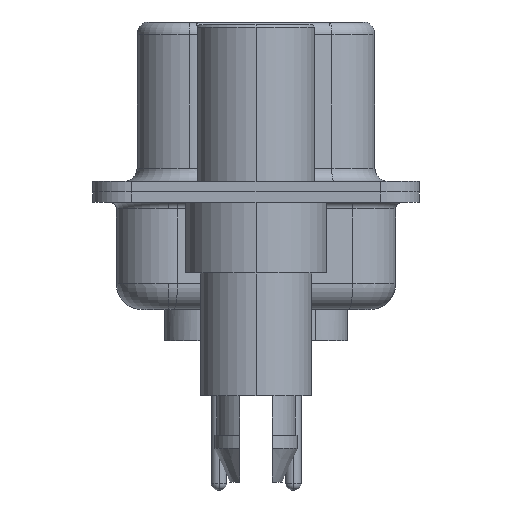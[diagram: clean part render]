
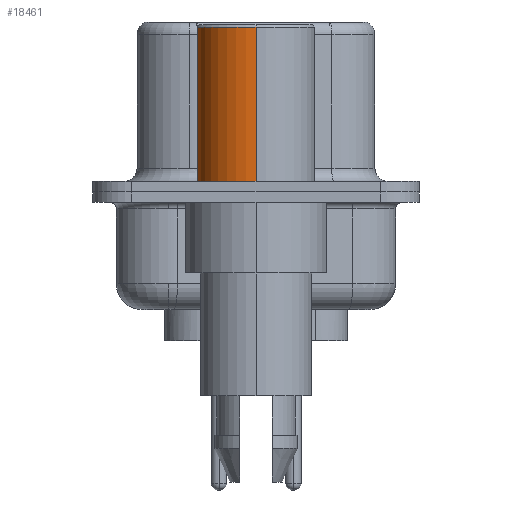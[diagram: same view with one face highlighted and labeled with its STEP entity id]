
A CAD part, left-side view. The second image highlights one B-rep face of the part: STEP entity #18461.
In plain terms, the highlighted cylindrical face has radius 2.25 mm (diameter 4.5 mm), a partial arc.
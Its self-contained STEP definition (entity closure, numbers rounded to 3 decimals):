
#1029 = VERTEX_POINT ( 'NONE', #7219 ) ;
#1498 = CARTESIAN_POINT ( 'NONE',  ( 2.25, 0., 0.581 ) ) ;
#1517 = ORIENTED_EDGE ( 'NONE', *, *, #14854, .F. ) ;
#1782 = CARTESIAN_POINT ( 'NONE',  ( -2.25, 0., 6.3 ) ) ;
#1797 = DIRECTION ( 'NONE',  ( 0., 0., 1. ) ) ;
#3846 = CARTESIAN_POINT ( 'NONE',  ( -2.25, 0., 0.581 ) ) ;
#4059 = AXIS2_PLACEMENT_3D ( 'NONE', #4210, #4727, #19889 ) ;
#4210 = CARTESIAN_POINT ( 'NONE',  ( 0., 0., 0.4 ) ) ;
#4727 = DIRECTION ( 'NONE',  ( 0., 0., 1. ) ) ;
#4913 = DIRECTION ( 'NONE',  ( 1., 0., 0. ) ) ;
#5925 = EDGE_LOOP ( 'NONE', ( #25306, #15087, #22395, #1517 ) ) ;
#6042 = DIRECTION ( 'NONE',  ( 0., 0., 1. ) ) ;
#6111 = CIRCLE ( 'NONE', #4059, 2.25 ) ;
#6275 = VERTEX_POINT ( 'NONE', #1782 ) ;
#6559 = VECTOR ( 'NONE', #9355, 1000. ) ;
#7219 = CARTESIAN_POINT ( 'NONE',  ( -2.25, 0., 0.4 ) ) ;
#7515 = EDGE_CURVE ( 'NONE', #22842, #1029, #6111, .T. ) ;
#7984 = AXIS2_PLACEMENT_3D ( 'NONE', #12091, #6042, #10286 ) ;
#9355 = DIRECTION ( 'NONE',  ( 0., 0., 1. ) ) ;
#10286 = DIRECTION ( 'NONE',  ( 1., 0., 0. ) ) ;
#10323 = DIRECTION ( 'NONE',  ( 0., 0., 1. ) ) ;
#11280 = LINE ( 'NONE', #1498, #6559 ) ;
#11818 = LINE ( 'NONE', #3846, #23378 ) ;
#12091 = CARTESIAN_POINT ( 'NONE',  ( 0., 0., 6.3 ) ) ;
#12632 = FACE_OUTER_BOUND ( 'NONE', #5925, .T. ) ;
#14072 = AXIS2_PLACEMENT_3D ( 'NONE', #22254, #10323, #4913 ) ;
#14374 = EDGE_CURVE ( 'NONE', #1029, #6275, #11818, .T. ) ;
#14854 = EDGE_CURVE ( 'NONE', #22842, #15048, #11280, .T. ) ;
#15013 = CARTESIAN_POINT ( 'NONE',  ( 2.25, 0., 0.4 ) ) ;
#15048 = VERTEX_POINT ( 'NONE', #24711 ) ;
#15087 = ORIENTED_EDGE ( 'NONE', *, *, #14374, .T. ) ;
#16605 = CIRCLE ( 'NONE', #7984, 2.25 ) ;
#18461 = ADVANCED_FACE ( 'NONE', ( #12632 ), #20573, .T. ) ;
#19889 = DIRECTION ( 'NONE',  ( 1., 0., 0. ) ) ;
#20573 = CYLINDRICAL_SURFACE ( 'NONE', #14072, 2.25 ) ;
#20705 = EDGE_CURVE ( 'NONE', #15048, #6275, #16605, .T. ) ;
#22254 = CARTESIAN_POINT ( 'NONE',  ( 0., 0., 0.581 ) ) ;
#22395 = ORIENTED_EDGE ( 'NONE', *, *, #20705, .F. ) ;
#22842 = VERTEX_POINT ( 'NONE', #15013 ) ;
#23378 = VECTOR ( 'NONE', #1797, 1000. ) ;
#24711 = CARTESIAN_POINT ( 'NONE',  ( 2.25, 0., 6.3 ) ) ;
#25306 = ORIENTED_EDGE ( 'NONE', *, *, #7515, .T. ) ;
